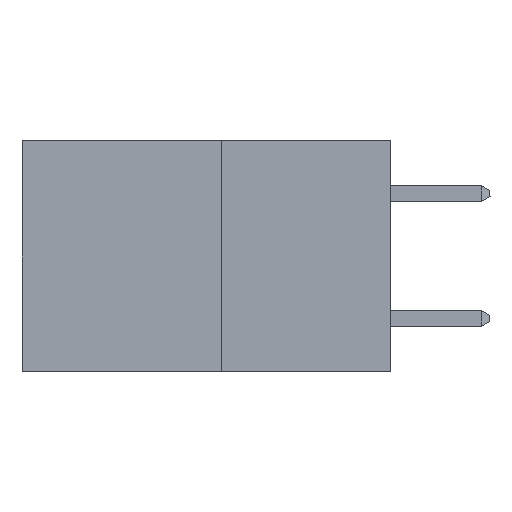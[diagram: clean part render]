
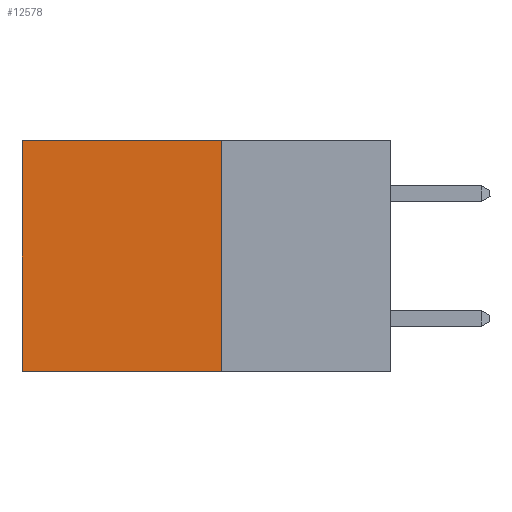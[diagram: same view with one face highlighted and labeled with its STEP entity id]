
A CAD part, left-side view. The second image highlights one B-rep face of the part: STEP entity #12578.
In plain terms, the highlighted planar face has unit normal (-1, 0, 0).
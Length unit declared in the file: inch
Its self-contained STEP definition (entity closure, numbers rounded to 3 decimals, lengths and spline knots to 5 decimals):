
#527 = AXIS2_PLACEMENT_3D ( 'NONE', #2545, #13327, #5329 ) ;
#987 = VECTOR ( 'NONE', #15367, 39.37008 ) ;
#1348 = VERTEX_POINT ( 'NONE', #11713 ) ;
#1499 = LINE ( 'NONE', #2338, #4747 ) ;
#1739 = CARTESIAN_POINT ( 'NONE',  ( 0.277, 0.27, 0. ) ) ;
#2195 = DIRECTION ( 'NONE',  ( 0., 0., -1. ) ) ;
#2338 = CARTESIAN_POINT ( 'NONE',  ( 0.277, 0.59, -0.37 ) ) ;
#2545 = CARTESIAN_POINT ( 'NONE',  ( 0.277, 0.27, -0.37 ) ) ;
#2717 = CARTESIAN_POINT ( 'NONE',  ( 0.277, 0.59, -0.37 ) ) ;
#4103 = CARTESIAN_POINT ( 'NONE',  ( 0.277, 0.27, -0.37 ) ) ;
#4189 = VERTEX_POINT ( 'NONE', #2717 ) ;
#4586 = ORIENTED_EDGE ( 'NONE', *, *, #7850, .T. ) ;
#4734 = LINE ( 'NONE', #10032, #14942 ) ;
#4747 = VECTOR ( 'NONE', #2195, 39.37008 ) ;
#5201 = ORIENTED_EDGE ( 'NONE', *, *, #5554, .F. ) ;
#5329 = DIRECTION ( 'NONE',  ( 0., 0., -1. ) ) ;
#5554 = EDGE_CURVE ( 'NONE', #14448, #14303, #11828, .T. ) ;
#6376 = FACE_OUTER_BOUND ( 'NONE', #6418, .T. ) ;
#6418 = EDGE_LOOP ( 'NONE', ( #4586, #12154, #5201, #16550 ) ) ;
#7850 = EDGE_CURVE ( 'NONE', #1348, #4189, #1499, .T. ) ;
#8271 = EDGE_CURVE ( 'NONE', #14303, #4189, #4734, .T. ) ;
#8967 = EDGE_CURVE ( 'NONE', #14448, #1348, #16502, .T. ) ;
#10032 = CARTESIAN_POINT ( 'NONE',  ( 0.277, 0.27, -0.37 ) ) ;
#10177 = DIRECTION ( 'NONE',  ( 0., 1., 0. ) ) ;
#11713 = CARTESIAN_POINT ( 'NONE',  ( 0.277, 0.59, 0. ) ) ;
#11828 = LINE ( 'NONE', #13242, #987 ) ;
#11999 = PLANE ( 'NONE',  #527 ) ;
#12154 = ORIENTED_EDGE ( 'NONE', *, *, #8271, .F. ) ;
#12242 = VECTOR ( 'NONE', #13720, 39.37008 ) ;
#12396 = CARTESIAN_POINT ( 'NONE',  ( 0.277, 0.27, 0. ) ) ;
#12578 = ADVANCED_FACE ( 'NONE', ( #6376 ), #11999, .F. ) ;
#13242 = CARTESIAN_POINT ( 'NONE',  ( 0.277, 0.27, -0.37 ) ) ;
#13327 = DIRECTION ( 'NONE',  ( 1., 0., 0. ) ) ;
#13720 = DIRECTION ( 'NONE',  ( 0., 1., 0. ) ) ;
#14303 = VERTEX_POINT ( 'NONE', #4103 ) ;
#14448 = VERTEX_POINT ( 'NONE', #1739 ) ;
#14942 = VECTOR ( 'NONE', #10177, 39.37008 ) ;
#15367 = DIRECTION ( 'NONE',  ( 0., 0., -1. ) ) ;
#16502 = LINE ( 'NONE', #12396, #12242 ) ;
#16550 = ORIENTED_EDGE ( 'NONE', *, *, #8967, .T. ) ;
